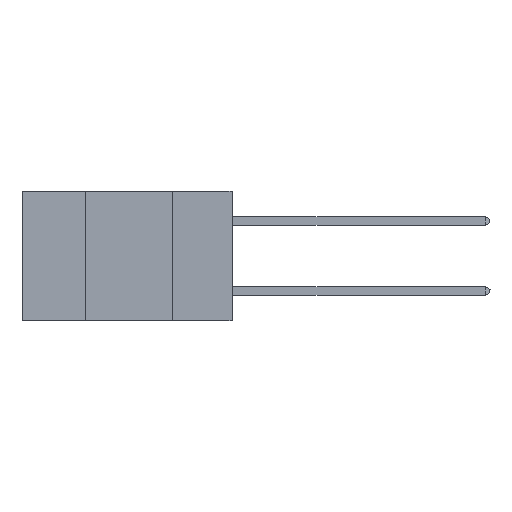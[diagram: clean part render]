
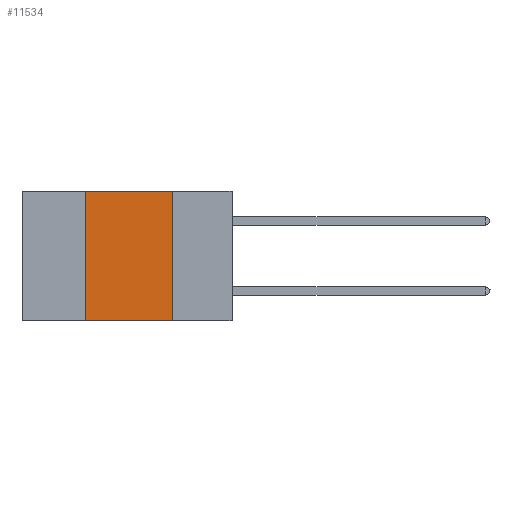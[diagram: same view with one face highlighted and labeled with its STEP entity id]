
A CAD part, left-side view. The second image highlights one B-rep face of the part: STEP entity #11534.
In plain terms, the highlighted planar face has unit normal (-1, 0, 0).
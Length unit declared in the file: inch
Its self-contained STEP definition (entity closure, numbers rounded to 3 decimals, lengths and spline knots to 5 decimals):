
#88 = VECTOR ( 'NONE', #5670, 39.37008 ) ;
#500 = PLANE ( 'NONE',  #3047 ) ;
#564 = EDGE_CURVE ( 'NONE', #25799, #1229, #22394, .T. ) ;
#575 = CARTESIAN_POINT ( 'NONE',  ( 0., 0.6, 0. ) ) ;
#726 = CARTESIAN_POINT ( 'NONE',  ( 0., 0.6, 0. ) ) ;
#852 = VERTEX_POINT ( 'NONE', #7445 ) ;
#1229 = VERTEX_POINT ( 'NONE', #12434 ) ;
#1661 = CARTESIAN_POINT ( 'NONE',  ( 0., 0.17, 0. ) ) ;
#1783 = ORIENTED_EDGE ( 'NONE', *, *, #11281, .F. ) ;
#3047 = AXIS2_PLACEMENT_3D ( 'NONE', #575, #12807, #14630 ) ;
#3065 = CARTESIAN_POINT ( 'NONE',  ( 0., 0.42, 0. ) ) ;
#3451 = VECTOR ( 'NONE', #13843, 39.37008 ) ;
#3727 = CARTESIAN_POINT ( 'NONE',  ( 0., 0.42, 0. ) ) ;
#5670 = DIRECTION ( 'NONE',  ( 0., 0., -1. ) ) ;
#6878 = LINE ( 'NONE', #3727, #3451 ) ;
#7445 = CARTESIAN_POINT ( 'NONE',  ( 0., 0.42, -0.37 ) ) ;
#7929 = DIRECTION ( 'NONE',  ( 0., -1., 0. ) ) ;
#8018 = CARTESIAN_POINT ( 'NONE',  ( 0., 0.6, -0.37 ) ) ;
#9370 = ORIENTED_EDGE ( 'NONE', *, *, #21810, .F. ) ;
#11281 = EDGE_CURVE ( 'NONE', #1229, #16343, #25044, .T. ) ;
#11356 = CARTESIAN_POINT ( 'NONE',  ( 0., 0.17, -0.37 ) ) ;
#11534 = ADVANCED_FACE ( 'NONE', ( #23155 ), #500, .F. ) ;
#11862 = VECTOR ( 'NONE', #7929, 39.37008 ) ;
#12434 = CARTESIAN_POINT ( 'NONE',  ( 0., 0.17, 0. ) ) ;
#12807 = DIRECTION ( 'NONE',  ( 1., 0., 0. ) ) ;
#13257 = ORIENTED_EDGE ( 'NONE', *, *, #564, .F. ) ;
#13843 = DIRECTION ( 'NONE',  ( 0., 0., 1. ) ) ;
#14630 = DIRECTION ( 'NONE',  ( 0., 0., -1. ) ) ;
#16343 = VERTEX_POINT ( 'NONE', #11356 ) ;
#20615 = DIRECTION ( 'NONE',  ( 0., -1., 0. ) ) ;
#21810 = EDGE_CURVE ( 'NONE', #852, #25799, #6878, .T. ) ;
#21843 = LINE ( 'NONE', #8018, #11862 ) ;
#22151 = EDGE_CURVE ( 'NONE', #852, #16343, #21843, .T. ) ;
#22394 = LINE ( 'NONE', #726, #25183 ) ;
#22709 = ORIENTED_EDGE ( 'NONE', *, *, #22151, .T. ) ;
#23155 = FACE_OUTER_BOUND ( 'NONE', #24883, .T. ) ;
#24883 = EDGE_LOOP ( 'NONE', ( #1783, #13257, #9370, #22709 ) ) ;
#25044 = LINE ( 'NONE', #1661, #88 ) ;
#25183 = VECTOR ( 'NONE', #20615, 39.37008 ) ;
#25799 = VERTEX_POINT ( 'NONE', #3065 ) ;
